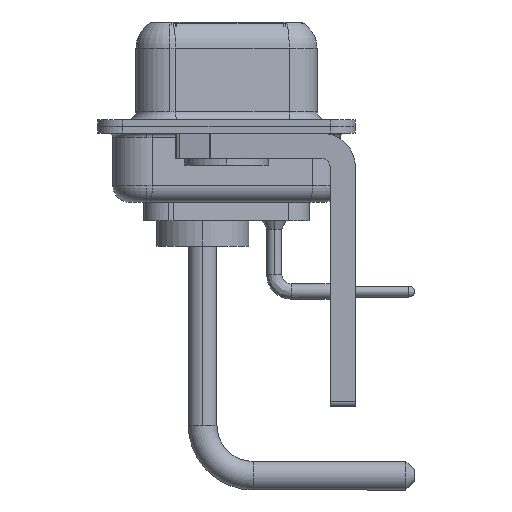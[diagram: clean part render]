
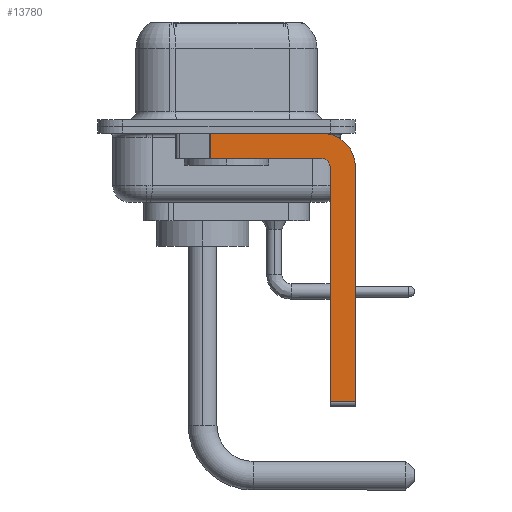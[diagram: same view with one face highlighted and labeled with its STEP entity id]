
A CAD part, left-side view. The second image highlights one B-rep face of the part: STEP entity #13780.
In plain terms, the highlighted planar face has unit normal (-1, 0, 0).
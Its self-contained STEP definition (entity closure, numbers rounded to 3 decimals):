
#356 = DIRECTION ( 'NONE',  ( 0., 0., -1. ) ) ;
#593 = AXIS2_PLACEMENT_3D ( 'NONE', #9756, #901, #16563 ) ;
#717 = CARTESIAN_POINT ( 'NONE',  ( -2.9, -5.65, -2.4 ) ) ;
#901 = DIRECTION ( 'NONE',  ( 1., 0., 0. ) ) ;
#1159 = VERTEX_POINT ( 'NONE', #21165 ) ;
#1261 = VECTOR ( 'NONE', #13946, 1000. ) ;
#1307 = EDGE_CURVE ( 'NONE', #15391, #1159, #4366, .T. ) ;
#1313 = CARTESIAN_POINT ( 'NONE',  ( -2.9, -7.65, -2.4 ) ) ;
#1436 = CARTESIAN_POINT ( 'NONE',  ( -2.9, 0.978, -0.4 ) ) ;
#2670 = EDGE_CURVE ( 'NONE', #15391, #7622, #7752, .T. ) ;
#2918 = DIRECTION ( 'NONE',  ( 0., 0., -1. ) ) ;
#3084 = CARTESIAN_POINT ( 'NONE',  ( -2.9, -5.65, -2.4 ) ) ;
#3428 = VECTOR ( 'NONE', #9523, 1000. ) ;
#3963 = CARTESIAN_POINT ( 'NONE',  ( -2.9, -5.65, -0.4 ) ) ;
#4366 = LINE ( 'NONE', #18266, #20969 ) ;
#4387 = CIRCLE ( 'NONE', #11825, 0.5 ) ;
#4468 = LINE ( 'NONE', #9788, #19978 ) ;
#4685 = DIRECTION ( 'NONE',  ( 0., 0., 1. ) ) ;
#5032 = CARTESIAN_POINT ( 'NONE',  ( -2.9, -7.65, -16.35 ) ) ;
#5963 = ORIENTED_EDGE ( 'NONE', *, *, #14344, .F. ) ;
#6298 = EDGE_CURVE ( 'NONE', #16888, #8476, #19026, .T. ) ;
#6933 = EDGE_CURVE ( 'NONE', #9006, #8476, #19551, .T. ) ;
#7219 = ORIENTED_EDGE ( 'NONE', *, *, #17436, .F. ) ;
#7295 = CIRCLE ( 'NONE', #593, 2. ) ;
#7458 = DIRECTION ( 'NONE',  ( -1., 0., 0. ) ) ;
#7536 = CARTESIAN_POINT ( 'NONE',  ( -2.9, -5.65, -16.35 ) ) ;
#7622 = VERTEX_POINT ( 'NONE', #5032 ) ;
#7752 = LINE ( 'NONE', #7536, #18822 ) ;
#8476 = VERTEX_POINT ( 'NONE', #11517 ) ;
#9006 = VERTEX_POINT ( 'NONE', #20389 ) ;
#9192 = CARTESIAN_POINT ( 'NONE',  ( -2.9, -5.65, -1.9 ) ) ;
#9510 = ORIENTED_EDGE ( 'NONE', *, *, #21340, .F. ) ;
#9523 = DIRECTION ( 'NONE',  ( 0., 1., 0. ) ) ;
#9756 = CARTESIAN_POINT ( 'NONE',  ( -2.9, -5.65, -2.4 ) ) ;
#9788 = CARTESIAN_POINT ( 'NONE',  ( -2.9, -7.65, -2.4 ) ) ;
#10419 = DIRECTION ( 'NONE',  ( 1., 0., 0. ) ) ;
#11069 = EDGE_LOOP ( 'NONE', ( #5963, #15386, #21936, #7219, #12585, #18959, #15219, #9510 ) ) ;
#11230 = VECTOR ( 'NONE', #356, 1000. ) ;
#11326 = DIRECTION ( 'NONE',  ( 0., -1., 0. ) ) ;
#11517 = CARTESIAN_POINT ( 'NONE',  ( -2.9, 0.978, -1.9 ) ) ;
#11825 = AXIS2_PLACEMENT_3D ( 'NONE', #717, #7458, #14261 ) ;
#12585 = ORIENTED_EDGE ( 'NONE', *, *, #1307, .F. ) ;
#12627 = EDGE_CURVE ( 'NONE', #20339, #7622, #4468, .T. ) ;
#13671 = PLANE ( 'NONE',  #21792 ) ;
#13780 = ADVANCED_FACE ( 'NONE', ( #18898 ), #13671, .F. ) ;
#13946 = DIRECTION ( 'NONE',  ( 0., -1., 0. ) ) ;
#14261 = DIRECTION ( 'NONE',  ( 0., 0., 1. ) ) ;
#14344 = EDGE_CURVE ( 'NONE', #16888, #15351, #19070, .T. ) ;
#15219 = ORIENTED_EDGE ( 'NONE', *, *, #12627, .F. ) ;
#15351 = VERTEX_POINT ( 'NONE', #3963 ) ;
#15386 = ORIENTED_EDGE ( 'NONE', *, *, #6298, .T. ) ;
#15391 = VERTEX_POINT ( 'NONE', #19861 ) ;
#16024 = CARTESIAN_POINT ( 'NONE',  ( -2.9, 0.978, -1.9 ) ) ;
#16067 = CARTESIAN_POINT ( 'NONE',  ( -2.9, 3., -0.4 ) ) ;
#16563 = DIRECTION ( 'NONE',  ( 0., 0., -1. ) ) ;
#16888 = VERTEX_POINT ( 'NONE', #1436 ) ;
#17436 = EDGE_CURVE ( 'NONE', #1159, #9006, #4387, .T. ) ;
#18266 = CARTESIAN_POINT ( 'NONE',  ( -2.9, -6.15, -16.6 ) ) ;
#18674 = DIRECTION ( 'NONE',  ( 0., 0., -1. ) ) ;
#18822 = VECTOR ( 'NONE', #11326, 1000. ) ;
#18898 = FACE_OUTER_BOUND ( 'NONE', #11069, .T. ) ;
#18959 = ORIENTED_EDGE ( 'NONE', *, *, #2670, .T. ) ;
#19026 = LINE ( 'NONE', #16024, #11230 ) ;
#19070 = LINE ( 'NONE', #16067, #1261 ) ;
#19551 = LINE ( 'NONE', #9192, #3428 ) ;
#19861 = CARTESIAN_POINT ( 'NONE',  ( -2.9, -6.15, -16.35 ) ) ;
#19978 = VECTOR ( 'NONE', #2918, 1000. ) ;
#20339 = VERTEX_POINT ( 'NONE', #1313 ) ;
#20389 = CARTESIAN_POINT ( 'NONE',  ( -2.9, -5.65, -1.9 ) ) ;
#20969 = VECTOR ( 'NONE', #4685, 1000. ) ;
#21165 = CARTESIAN_POINT ( 'NONE',  ( -2.9, -6.15, -2.4 ) ) ;
#21340 = EDGE_CURVE ( 'NONE', #15351, #20339, #7295, .T. ) ;
#21792 = AXIS2_PLACEMENT_3D ( 'NONE', #3084, #10419, #18674 ) ;
#21936 = ORIENTED_EDGE ( 'NONE', *, *, #6933, .F. ) ;
